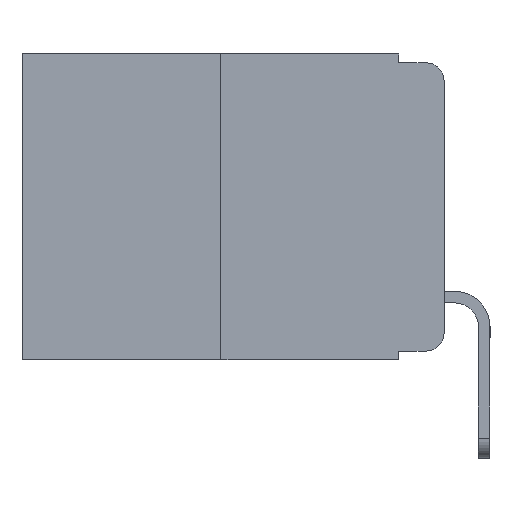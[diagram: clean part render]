
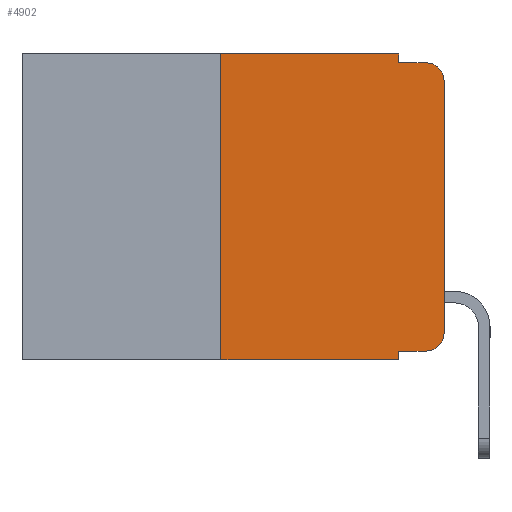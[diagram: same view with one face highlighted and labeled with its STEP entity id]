
A CAD part, left-side view. The second image highlights one B-rep face of the part: STEP entity #4902.
In plain terms, the highlighted planar face has unit normal (-1, 0, 0).
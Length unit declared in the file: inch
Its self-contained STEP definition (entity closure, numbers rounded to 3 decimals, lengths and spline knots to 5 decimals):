
#89 = LINE ( 'NONE', #7437, #9820 ) ;
#165 = LINE ( 'NONE', #13885, #3353 ) ;
#411 = EDGE_CURVE ( 'NONE', #4408, #13818, #13969, .T. ) ;
#650 = CARTESIAN_POINT ( 'NONE',  ( 0., 0.25, 0. ) ) ;
#1337 = VERTEX_POINT ( 'NONE', #3415 ) ;
#1350 = VERTEX_POINT ( 'NONE', #13908 ) ;
#1587 = VERTEX_POINT ( 'NONE', #3115 ) ;
#2041 = ORIENTED_EDGE ( 'NONE', *, *, #7729, .F. ) ;
#2176 = LINE ( 'NONE', #11444, #14573 ) ;
#2576 = ORIENTED_EDGE ( 'NONE', *, *, #15081, .T. ) ;
#2908 = ORIENTED_EDGE ( 'NONE', *, *, #4108, .T. ) ;
#3115 = CARTESIAN_POINT ( 'NONE',  ( 0., 0.02, -0.01 ) ) ;
#3150 = ORIENTED_EDGE ( 'NONE', *, *, #411, .F. ) ;
#3353 = VECTOR ( 'NONE', #7218, 39.37008 ) ;
#3409 = ORIENTED_EDGE ( 'NONE', *, *, #6486, .T. ) ;
#3415 = CARTESIAN_POINT ( 'NONE',  ( 0., 0.051, -0.01 ) ) ;
#3425 = DIRECTION ( 'NONE',  ( -1., 0., 0. ) ) ;
#3478 = CARTESIAN_POINT ( 'NONE',  ( 0., 0.051, 0. ) ) ;
#3538 = VERTEX_POINT ( 'NONE', #3478 ) ;
#3932 = CARTESIAN_POINT ( 'NONE',  ( 0., 0.473, 0. ) ) ;
#3975 = DIRECTION ( 'NONE',  ( 0., -1., 0. ) ) ;
#4108 = EDGE_CURVE ( 'NONE', #4408, #8026, #2176, .T. ) ;
#4224 = DIRECTION ( 'NONE',  ( -1., 0., 0. ) ) ;
#4408 = VERTEX_POINT ( 'NONE', #7022 ) ;
#4516 = VECTOR ( 'NONE', #5478, 39.37008 ) ;
#4902 = ADVANCED_FACE ( 'NONE', ( #5429 ), #12601, .F. ) ;
#5338 = DIRECTION ( 'NONE',  ( 0., -1., 0. ) ) ;
#5429 = FACE_OUTER_BOUND ( 'NONE', #12631, .T. ) ;
#5451 = ORIENTED_EDGE ( 'NONE', *, *, #12817, .T. ) ;
#5464 = LINE ( 'NONE', #14734, #11457 ) ;
#5478 = DIRECTION ( 'NONE',  ( 0., 0., -1. ) ) ;
#5639 = ORIENTED_EDGE ( 'NONE', *, *, #7941, .T. ) ;
#5713 = LINE ( 'NONE', #7972, #14950 ) ;
#6140 = VERTEX_POINT ( 'NONE', #14765 ) ;
#6218 = CARTESIAN_POINT ( 'NONE',  ( 0., 0.02, -0.333 ) ) ;
#6413 = VERTEX_POINT ( 'NONE', #8763 ) ;
#6486 = EDGE_CURVE ( 'NONE', #6413, #13818, #10856, .T. ) ;
#7022 = CARTESIAN_POINT ( 'NONE',  ( 0., 0.051, -0.333 ) ) ;
#7178 = AXIS2_PLACEMENT_3D ( 'NONE', #11467, #4224, #12597 ) ;
#7218 = DIRECTION ( 'NONE',  ( 0., -1., 0. ) ) ;
#7301 = CARTESIAN_POINT ( 'NONE',  ( 0., 0.051, -0.343 ) ) ;
#7411 = DIRECTION ( 'NONE',  ( 0., 0., 1. ) ) ;
#7437 = CARTESIAN_POINT ( 'NONE',  ( 0., 0.25, 0. ) ) ;
#7637 = CIRCLE ( 'NONE', #10471, 0.02 ) ;
#7696 = VECTOR ( 'NONE', #5338, 39.37008 ) ;
#7719 = CARTESIAN_POINT ( 'NONE',  ( 0., 0.473, -0.343 ) ) ;
#7729 = EDGE_CURVE ( 'NONE', #1337, #1587, #165, .T. ) ;
#7941 = EDGE_CURVE ( 'NONE', #6140, #1350, #5713, .T. ) ;
#7972 = CARTESIAN_POINT ( 'NONE',  ( 0., 0., 0. ) ) ;
#8026 = VERTEX_POINT ( 'NONE', #6218 ) ;
#8213 = ORIENTED_EDGE ( 'NONE', *, *, #14891, .F. ) ;
#8333 = ORIENTED_EDGE ( 'NONE', *, *, #10541, .F. ) ;
#8606 = ORIENTED_EDGE ( 'NONE', *, *, #8746, .F. ) ;
#8746 = EDGE_CURVE ( 'NONE', #3538, #1337, #5464, .T. ) ;
#8763 = CARTESIAN_POINT ( 'NONE',  ( 0., 0.25, -0.343 ) ) ;
#9228 = DIRECTION ( 'NONE',  ( 0., 0., -1. ) ) ;
#9285 = CARTESIAN_POINT ( 'NONE',  ( 0., 0.473, 0. ) ) ;
#9782 = LINE ( 'NONE', #3932, #15344 ) ;
#9820 = VECTOR ( 'NONE', #11023, 39.37008 ) ;
#9948 = DIRECTION ( 'NONE',  ( 0., -1., 0. ) ) ;
#10471 = AXIS2_PLACEMENT_3D ( 'NONE', #10732, #3425, #11895 ) ;
#10541 = EDGE_CURVE ( 'NONE', #14235, #3538, #9782, .T. ) ;
#10715 = DIRECTION ( 'NONE',  ( 0., 0., -1. ) ) ;
#10732 = CARTESIAN_POINT ( 'NONE',  ( 0., 0.02, -0.03 ) ) ;
#10856 = LINE ( 'NONE', #7719, #7696 ) ;
#11023 = DIRECTION ( 'NONE',  ( 0., 0., 1. ) ) ;
#11444 = CARTESIAN_POINT ( 'NONE',  ( 0., 0.051, -0.333 ) ) ;
#11457 = VECTOR ( 'NONE', #9228, 39.37008 ) ;
#11467 = CARTESIAN_POINT ( 'NONE',  ( 0., 0.02, -0.313 ) ) ;
#11895 = DIRECTION ( 'NONE',  ( 0., 0., -1. ) ) ;
#12597 = DIRECTION ( 'NONE',  ( 0., 0., -1. ) ) ;
#12601 = PLANE ( 'NONE',  #14001 ) ;
#12631 = EDGE_LOOP ( 'NONE', ( #5639, #5451, #2041, #8606, #8333, #8213, #3409, #3150, #2908, #2576 ) ) ;
#12817 = EDGE_CURVE ( 'NONE', #1350, #1587, #7637, .T. ) ;
#13818 = VERTEX_POINT ( 'NONE', #7301 ) ;
#13885 = CARTESIAN_POINT ( 'NONE',  ( 0., 0.051, -0.01 ) ) ;
#13908 = CARTESIAN_POINT ( 'NONE',  ( 0., 0., -0.03 ) ) ;
#13969 = LINE ( 'NONE', #15530, #4516 ) ;
#14001 = AXIS2_PLACEMENT_3D ( 'NONE', #9285, #14108, #10715 ) ;
#14108 = DIRECTION ( 'NONE',  ( 1., 0., 0. ) ) ;
#14235 = VERTEX_POINT ( 'NONE', #650 ) ;
#14573 = VECTOR ( 'NONE', #9948, 39.37008 ) ;
#14734 = CARTESIAN_POINT ( 'NONE',  ( 0., 0.051, 0. ) ) ;
#14765 = CARTESIAN_POINT ( 'NONE',  ( 0., 0., -0.313 ) ) ;
#14891 = EDGE_CURVE ( 'NONE', #6413, #14235, #89, .T. ) ;
#14950 = VECTOR ( 'NONE', #7411, 39.37008 ) ;
#15081 = EDGE_CURVE ( 'NONE', #8026, #6140, #15225, .T. ) ;
#15225 = CIRCLE ( 'NONE', #7178, 0.02 ) ;
#15344 = VECTOR ( 'NONE', #3975, 39.37008 ) ;
#15530 = CARTESIAN_POINT ( 'NONE',  ( 0., 0.051, 0. ) ) ;
